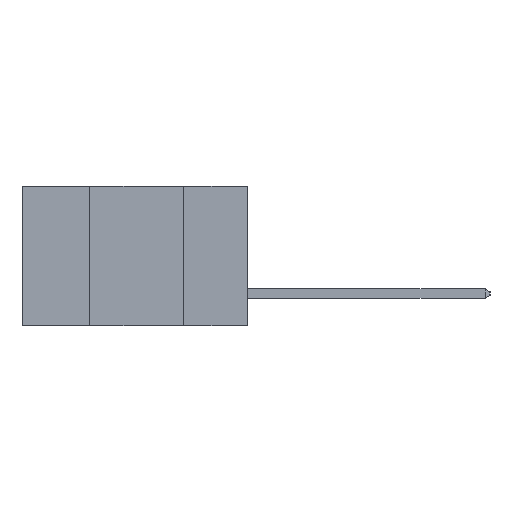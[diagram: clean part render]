
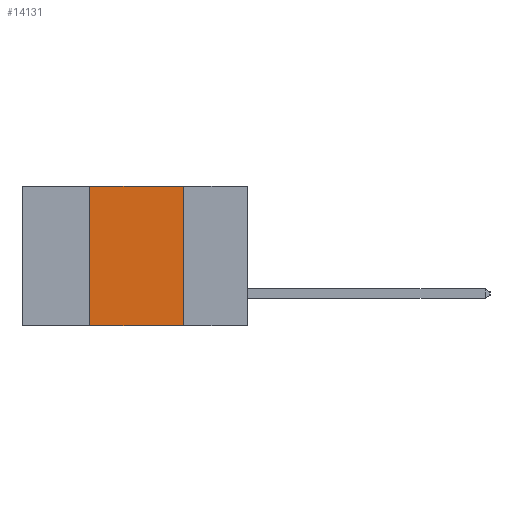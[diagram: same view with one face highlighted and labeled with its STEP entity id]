
A CAD part, left-side view. The second image highlights one B-rep face of the part: STEP entity #14131.
In plain terms, the highlighted planar face has unit normal (-1, 0, 0).
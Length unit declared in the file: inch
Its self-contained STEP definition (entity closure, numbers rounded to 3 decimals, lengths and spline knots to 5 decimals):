
#351 = CARTESIAN_POINT ( 'NONE',  ( 0., 0.42, 0. ) ) ;
#466 = EDGE_CURVE ( 'NONE', #9224, #11538, #8695, .T. ) ;
#611 = CARTESIAN_POINT ( 'NONE',  ( 0., 0.6, 0. ) ) ;
#832 = VECTOR ( 'NONE', #7533, 39.37008 ) ;
#1399 = AXIS2_PLACEMENT_3D ( 'NONE', #2655, #4898, #14281 ) ;
#1505 = EDGE_LOOP ( 'NONE', ( #6380, #7637, #12360, #5248 ) ) ;
#2609 = PLANE ( 'NONE',  #1399 ) ;
#2655 = CARTESIAN_POINT ( 'NONE',  ( 0., 0.6, 0. ) ) ;
#2720 = CARTESIAN_POINT ( 'NONE',  ( 0., 0.17, 0. ) ) ;
#3323 = VERTEX_POINT ( 'NONE', #2720 ) ;
#3939 = DIRECTION ( 'NONE',  ( 0., -1., 0. ) ) ;
#4085 = CARTESIAN_POINT ( 'NONE',  ( 0., 0.42, -0.37 ) ) ;
#4334 = EDGE_CURVE ( 'NONE', #3323, #10269, #8590, .T. ) ;
#4518 = EDGE_CURVE ( 'NONE', #11538, #3323, #7831, .T. ) ;
#4695 = LINE ( 'NONE', #11840, #12640 ) ;
#4898 = DIRECTION ( 'NONE',  ( 1., 0., 0. ) ) ;
#5218 = FACE_OUTER_BOUND ( 'NONE', #1505, .T. ) ;
#5248 = ORIENTED_EDGE ( 'NONE', *, *, #14461, .T. ) ;
#5386 = CARTESIAN_POINT ( 'NONE',  ( 0., 0.17, -0.37 ) ) ;
#5821 = CARTESIAN_POINT ( 'NONE',  ( 0., 0.17, -0.37 ) ) ;
#6380 = ORIENTED_EDGE ( 'NONE', *, *, #4334, .F. ) ;
#6577 = VECTOR ( 'NONE', #3939, 39.37008 ) ;
#7533 = DIRECTION ( 'NONE',  ( 0., 0., -1. ) ) ;
#7637 = ORIENTED_EDGE ( 'NONE', *, *, #4518, .F. ) ;
#7831 = LINE ( 'NONE', #611, #6577 ) ;
#8590 = LINE ( 'NONE', #5386, #832 ) ;
#8695 = LINE ( 'NONE', #4085, #11046 ) ;
#9224 = VERTEX_POINT ( 'NONE', #9233 ) ;
#9233 = CARTESIAN_POINT ( 'NONE',  ( 0., 0.42, -0.37 ) ) ;
#10269 = VERTEX_POINT ( 'NONE', #5821 ) ;
#11046 = VECTOR ( 'NONE', #14547, 39.37008 ) ;
#11538 = VERTEX_POINT ( 'NONE', #351 ) ;
#11840 = CARTESIAN_POINT ( 'NONE',  ( 0., 0.6, -0.37 ) ) ;
#12360 = ORIENTED_EDGE ( 'NONE', *, *, #466, .F. ) ;
#12371 = DIRECTION ( 'NONE',  ( 0., -1., 0. ) ) ;
#12640 = VECTOR ( 'NONE', #12371, 39.37008 ) ;
#14131 = ADVANCED_FACE ( 'NONE', ( #5218 ), #2609, .F. ) ;
#14281 = DIRECTION ( 'NONE',  ( 0., 0., -1. ) ) ;
#14461 = EDGE_CURVE ( 'NONE', #9224, #10269, #4695, .T. ) ;
#14547 = DIRECTION ( 'NONE',  ( 0., 0., 1. ) ) ;
